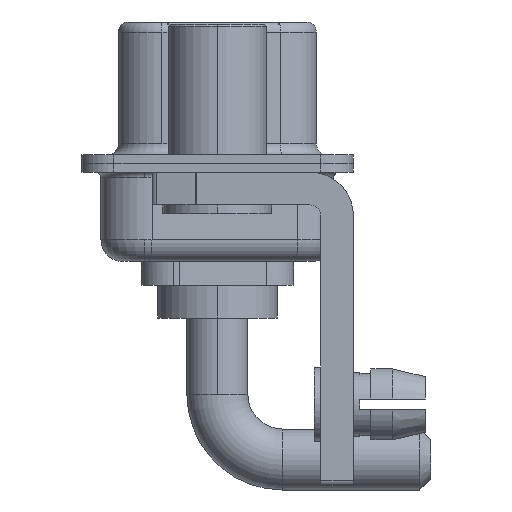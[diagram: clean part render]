
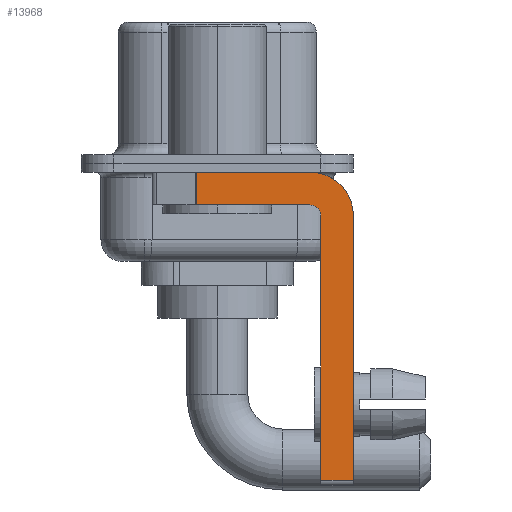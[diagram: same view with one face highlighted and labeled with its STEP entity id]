
A CAD part, left-side view. The second image highlights one B-rep face of the part: STEP entity #13968.
In plain terms, the highlighted planar face has unit normal (-1, 0, 0).
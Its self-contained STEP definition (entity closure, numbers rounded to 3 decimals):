
#2 = EDGE_CURVE ( 'NONE', #19804, #6659, #10375, .T. ) ;
#393 = DIRECTION ( 'NONE',  ( 1., 0., 0. ) ) ;
#1214 = LINE ( 'NONE', #15615, #3388 ) ;
#1326 = EDGE_CURVE ( 'NONE', #2518, #1723, #18781, .T. ) ;
#1329 = CARTESIAN_POINT ( 'NONE',  ( -2.9, -4.75, -2.4 ) ) ;
#1723 = VERTEX_POINT ( 'NONE', #1981 ) ;
#1893 = ORIENTED_EDGE ( 'NONE', *, *, #4407, .F. ) ;
#1981 = CARTESIAN_POINT ( 'NONE',  ( -2.9, -4.25, -1.9 ) ) ;
#2518 = VERTEX_POINT ( 'NONE', #1329 ) ;
#2692 = DIRECTION ( 'NONE',  ( 1., 0., 0. ) ) ;
#2915 = LINE ( 'NONE', #9132, #19154 ) ;
#2922 = ORIENTED_EDGE ( 'NONE', *, *, #1326, .F. ) ;
#3388 = VECTOR ( 'NONE', #7519, 1000. ) ;
#3391 = AXIS2_PLACEMENT_3D ( 'NONE', #8818, #12214, #7475 ) ;
#3546 = PLANE ( 'NONE',  #10133 ) ;
#3631 = CARTESIAN_POINT ( 'NONE',  ( -2.9, -4.75, -14.8 ) ) ;
#3675 = CARTESIAN_POINT ( 'NONE',  ( -2.9, -6.25, -14.55 ) ) ;
#4024 = VECTOR ( 'NONE', #19424, 1000. ) ;
#4407 = EDGE_CURVE ( 'NONE', #9515, #10182, #7481, .T. ) ;
#4686 = FACE_OUTER_BOUND ( 'NONE', #16120, .T. ) ;
#5190 = ORIENTED_EDGE ( 'NONE', *, *, #19732, .F. ) ;
#5439 = EDGE_CURVE ( 'NONE', #10182, #6659, #1214, .T. ) ;
#5535 = DIRECTION ( 'NONE',  ( 0., 0., -1. ) ) ;
#6032 = DIRECTION ( 'NONE',  ( 0., -1., 0. ) ) ;
#6176 = CARTESIAN_POINT ( 'NONE',  ( -2.9, -4.25, -1.9 ) ) ;
#6594 = CARTESIAN_POINT ( 'NONE',  ( -2.9, -4.25, -2.4 ) ) ;
#6659 = VERTEX_POINT ( 'NONE', #3675 ) ;
#7475 = DIRECTION ( 'NONE',  ( 0., 0., 1. ) ) ;
#7481 = CIRCLE ( 'NONE', #10129, 2. ) ;
#7519 = DIRECTION ( 'NONE',  ( 0., 0., -1. ) ) ;
#8818 = CARTESIAN_POINT ( 'NONE',  ( -2.9, -4.25, -2.4 ) ) ;
#9132 = CARTESIAN_POINT ( 'NONE',  ( -2.9, 3., -0.4 ) ) ;
#9515 = VERTEX_POINT ( 'NONE', #10965 ) ;
#9922 = VECTOR ( 'NONE', #18609, 1000. ) ;
#9988 = VERTEX_POINT ( 'NONE', #14549 ) ;
#10129 = AXIS2_PLACEMENT_3D ( 'NONE', #16701, #2692, #5535 ) ;
#10133 = AXIS2_PLACEMENT_3D ( 'NONE', #6594, #393, #10927 ) ;
#10182 = VERTEX_POINT ( 'NONE', #16582 ) ;
#10375 = LINE ( 'NONE', #14033, #15789 ) ;
#10811 = LINE ( 'NONE', #6176, #9922 ) ;
#10927 = DIRECTION ( 'NONE',  ( 0., 0., -1. ) ) ;
#10965 = CARTESIAN_POINT ( 'NONE',  ( -2.9, -4.25, -0.4 ) ) ;
#11111 = CARTESIAN_POINT ( 'NONE',  ( -2.9, -4.75, -14.55 ) ) ;
#12214 = DIRECTION ( 'NONE',  ( -1., 0., 0. ) ) ;
#12918 = LINE ( 'NONE', #13021, #16734 ) ;
#13021 = CARTESIAN_POINT ( 'NONE',  ( -2.9, 0.978, -1.9 ) ) ;
#13697 = ORIENTED_EDGE ( 'NONE', *, *, #20188, .F. ) ;
#13968 = ADVANCED_FACE ( 'NONE', ( #4686 ), #3546, .F. ) ;
#14033 = CARTESIAN_POINT ( 'NONE',  ( -2.9, -4.25, -14.55 ) ) ;
#14549 = CARTESIAN_POINT ( 'NONE',  ( -2.9, 0.978, -0.4 ) ) ;
#14916 = ORIENTED_EDGE ( 'NONE', *, *, #18269, .T. ) ;
#15615 = CARTESIAN_POINT ( 'NONE',  ( -2.9, -6.25, -2.4 ) ) ;
#15789 = VECTOR ( 'NONE', #6032, 1000. ) ;
#16110 = LINE ( 'NONE', #3631, #4024 ) ;
#16120 = EDGE_LOOP ( 'NONE', ( #13697, #14916, #5190, #2922, #17480, #17315, #17132, #1893 ) ) ;
#16582 = CARTESIAN_POINT ( 'NONE',  ( -2.9, -6.25, -2.4 ) ) ;
#16701 = CARTESIAN_POINT ( 'NONE',  ( -2.9, -4.25, -2.4 ) ) ;
#16734 = VECTOR ( 'NONE', #17541, 1000. ) ;
#17132 = ORIENTED_EDGE ( 'NONE', *, *, #5439, .F. ) ;
#17312 = EDGE_CURVE ( 'NONE', #19804, #2518, #16110, .T. ) ;
#17315 = ORIENTED_EDGE ( 'NONE', *, *, #2, .T. ) ;
#17480 = ORIENTED_EDGE ( 'NONE', *, *, #17312, .F. ) ;
#17541 = DIRECTION ( 'NONE',  ( 0., 0., -1. ) ) ;
#18269 = EDGE_CURVE ( 'NONE', #9988, #19778, #12918, .T. ) ;
#18308 = CARTESIAN_POINT ( 'NONE',  ( -2.9, 0.978, -1.9 ) ) ;
#18609 = DIRECTION ( 'NONE',  ( 0., 1., 0. ) ) ;
#18781 = CIRCLE ( 'NONE', #3391, 0.5 ) ;
#19154 = VECTOR ( 'NONE', #19819, 1000. ) ;
#19424 = DIRECTION ( 'NONE',  ( 0., 0., 1. ) ) ;
#19732 = EDGE_CURVE ( 'NONE', #1723, #19778, #10811, .T. ) ;
#19778 = VERTEX_POINT ( 'NONE', #18308 ) ;
#19804 = VERTEX_POINT ( 'NONE', #11111 ) ;
#19819 = DIRECTION ( 'NONE',  ( 0., -1., 0. ) ) ;
#20188 = EDGE_CURVE ( 'NONE', #9988, #9515, #2915, .T. ) ;
